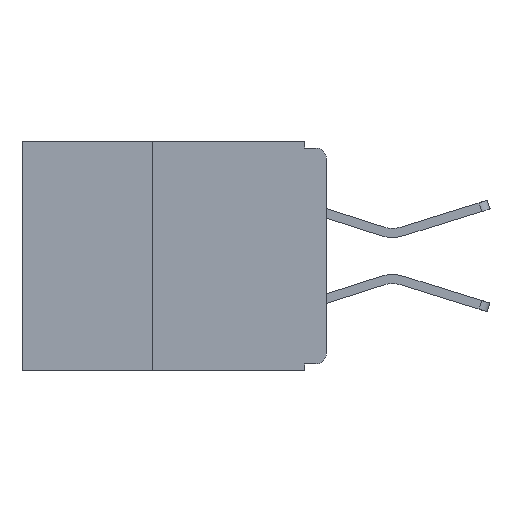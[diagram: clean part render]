
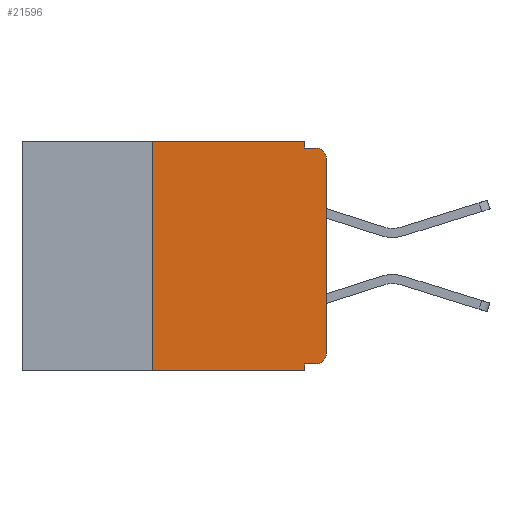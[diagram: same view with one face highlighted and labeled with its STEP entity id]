
A CAD part, left-side view. The second image highlights one B-rep face of the part: STEP entity #21596.
In plain terms, the highlighted planar face has unit normal (-1, 0, 0).
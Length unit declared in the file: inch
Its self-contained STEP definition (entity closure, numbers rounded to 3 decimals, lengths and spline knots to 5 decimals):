
#235 = VERTEX_POINT ( 'NONE', #23356 ) ;
#507 = CARTESIAN_POINT ( 'NONE',  ( 0., 0.25, 0. ) ) ;
#728 = CIRCLE ( 'NONE', #20448, 0.015 ) ;
#1158 = DIRECTION ( 'NONE',  ( 0., 0., 1. ) ) ;
#1184 = DIRECTION ( 'NONE',  ( 0., 0., -1. ) ) ;
#2012 = CARTESIAN_POINT ( 'NONE',  ( 0., 0.031, -0.33 ) ) ;
#2668 = LINE ( 'NONE', #7204, #6697 ) ;
#2838 = EDGE_CURVE ( 'NONE', #235, #18373, #9564, .T. ) ;
#3641 = EDGE_CURVE ( 'NONE', #5567, #24492, #22565, .T. ) ;
#3688 = DIRECTION ( 'NONE',  ( 0., -1., 0. ) ) ;
#3811 = CARTESIAN_POINT ( 'NONE',  ( 0., 0.031, -0.01 ) ) ;
#4426 = CARTESIAN_POINT ( 'NONE',  ( 0., 0.437, 0. ) ) ;
#4530 = EDGE_LOOP ( 'NONE', ( #5044, #5213, #5496, #6516, #8083, #8363, #9091, #9255, #10187, #10732 ) ) ;
#4605 = CARTESIAN_POINT ( 'NONE',  ( 0., 0.031, -0.32 ) ) ;
#4808 = VECTOR ( 'NONE', #1158, 39.37008 ) ;
#5044 = ORIENTED_EDGE ( 'NONE', *, *, #21000, .T. ) ;
#5213 = ORIENTED_EDGE ( 'NONE', *, *, #3641, .T. ) ;
#5278 = DIRECTION ( 'NONE',  ( 0., 0., 1. ) ) ;
#5452 = CARTESIAN_POINT ( 'NONE',  ( 0., 0.25, -0.33 ) ) ;
#5496 = ORIENTED_EDGE ( 'NONE', *, *, #11283, .F. ) ;
#5567 = VERTEX_POINT ( 'NONE', #8729 ) ;
#5871 = VECTOR ( 'NONE', #16764, 39.37008 ) ;
#6180 = VERTEX_POINT ( 'NONE', #5452 ) ;
#6516 = ORIENTED_EDGE ( 'NONE', *, *, #2838, .F. ) ;
#6697 = VECTOR ( 'NONE', #5278, 39.37008 ) ;
#7054 = EDGE_CURVE ( 'NONE', #16185, #235, #16414, .T. ) ;
#7091 = DIRECTION ( 'NONE',  ( 0., 0., -1. ) ) ;
#7123 = DIRECTION ( 'NONE',  ( -1., 0., 0. ) ) ;
#7169 = CARTESIAN_POINT ( 'NONE',  ( 0., 0.015, -0.025 ) ) ;
#7204 = CARTESIAN_POINT ( 'NONE',  ( 0., 0.25, -0.33 ) ) ;
#7321 = EDGE_CURVE ( 'NONE', #6180, #15299, #14860, .T. ) ;
#7912 = EDGE_CURVE ( 'NONE', #21474, #18129, #11179, .T. ) ;
#8013 = EDGE_CURVE ( 'NONE', #18129, #15299, #8695, .T. ) ;
#8066 = DIRECTION ( 'NONE',  ( 0., -1., 0. ) ) ;
#8083 = ORIENTED_EDGE ( 'NONE', *, *, #7054, .F. ) ;
#8130 = CARTESIAN_POINT ( 'NONE',  ( 0., 0.015, -0.01 ) ) ;
#8363 = ORIENTED_EDGE ( 'NONE', *, *, #17548, .F. ) ;
#8695 = LINE ( 'NONE', #15451, #9328 ) ;
#8729 = CARTESIAN_POINT ( 'NONE',  ( 0., 0., -0.025 ) ) ;
#8743 = CARTESIAN_POINT ( 'NONE',  ( 0., 0., -0.305 ) ) ;
#9091 = ORIENTED_EDGE ( 'NONE', *, *, #7321, .T. ) ;
#9255 = ORIENTED_EDGE ( 'NONE', *, *, #8013, .F. ) ;
#9328 = VECTOR ( 'NONE', #15723, 39.37008 ) ;
#9564 = LINE ( 'NONE', #16830, #19241 ) ;
#9667 = VECTOR ( 'NONE', #23310, 39.37008 ) ;
#10187 = ORIENTED_EDGE ( 'NONE', *, *, #7912, .F. ) ;
#10609 = VECTOR ( 'NONE', #3688, 39.37008 ) ;
#10732 = ORIENTED_EDGE ( 'NONE', *, *, #22317, .T. ) ;
#10925 = DIRECTION ( 'NONE',  ( 1., 0., 0. ) ) ;
#11179 = LINE ( 'NONE', #16911, #5871 ) ;
#11283 = EDGE_CURVE ( 'NONE', #18373, #24492, #15090, .T. ) ;
#13033 = DIRECTION ( 'NONE',  ( -1., 0., 0. ) ) ;
#14860 = LINE ( 'NONE', #23315, #9667 ) ;
#15090 = LINE ( 'NONE', #19697, #24043 ) ;
#15299 = VERTEX_POINT ( 'NONE', #2012 ) ;
#15451 = CARTESIAN_POINT ( 'NONE',  ( 0., 0.031, -0.33 ) ) ;
#15723 = DIRECTION ( 'NONE',  ( 0., 0., -1. ) ) ;
#16185 = VERTEX_POINT ( 'NONE', #507 ) ;
#16248 = VERTEX_POINT ( 'NONE', #8743 ) ;
#16291 = AXIS2_PLACEMENT_3D ( 'NONE', #20539, #10925, #24363 ) ;
#16414 = LINE ( 'NONE', #4426, #10609 ) ;
#16723 = PLANE ( 'NONE',  #16291 ) ;
#16764 = DIRECTION ( 'NONE',  ( 0., 1., 0. ) ) ;
#16765 = DIRECTION ( 'NONE',  ( 0., 0., -1. ) ) ;
#16830 = CARTESIAN_POINT ( 'NONE',  ( 0., 0.031, 0. ) ) ;
#16911 = CARTESIAN_POINT ( 'NONE',  ( 0., 0., -0.32 ) ) ;
#17548 = EDGE_CURVE ( 'NONE', #6180, #16185, #2668, .T. ) ;
#18129 = VERTEX_POINT ( 'NONE', #4605 ) ;
#18373 = VERTEX_POINT ( 'NONE', #3811 ) ;
#19241 = VECTOR ( 'NONE', #16765, 39.37008 ) ;
#19697 = CARTESIAN_POINT ( 'NONE',  ( 0., 0., -0.01 ) ) ;
#20210 = CARTESIAN_POINT ( 'NONE',  ( 0., 0.015, -0.32 ) ) ;
#20384 = LINE ( 'NONE', #22589, #4808 ) ;
#20448 = AXIS2_PLACEMENT_3D ( 'NONE', #24491, #13033, #1184 ) ;
#20539 = CARTESIAN_POINT ( 'NONE',  ( 0., 0.437, 0. ) ) ;
#21000 = EDGE_CURVE ( 'NONE', #16248, #5567, #20384, .T. ) ;
#21080 = AXIS2_PLACEMENT_3D ( 'NONE', #7169, #7123, #7091 ) ;
#21474 = VERTEX_POINT ( 'NONE', #20210 ) ;
#21596 = ADVANCED_FACE ( 'NONE', ( #21857 ), #16723, .F. ) ;
#21857 = FACE_OUTER_BOUND ( 'NONE', #4530, .T. ) ;
#22317 = EDGE_CURVE ( 'NONE', #21474, #16248, #728, .T. ) ;
#22565 = CIRCLE ( 'NONE', #21080, 0.015 ) ;
#22589 = CARTESIAN_POINT ( 'NONE',  ( 0., 0., 0. ) ) ;
#23310 = DIRECTION ( 'NONE',  ( 0., -1., 0. ) ) ;
#23315 = CARTESIAN_POINT ( 'NONE',  ( 0., 0.437, -0.33 ) ) ;
#23356 = CARTESIAN_POINT ( 'NONE',  ( 0., 0.031, 0. ) ) ;
#24043 = VECTOR ( 'NONE', #8066, 39.37008 ) ;
#24363 = DIRECTION ( 'NONE',  ( 0., 0., -1. ) ) ;
#24491 = CARTESIAN_POINT ( 'NONE',  ( 0., 0.015, -0.305 ) ) ;
#24492 = VERTEX_POINT ( 'NONE', #8130 ) ;
